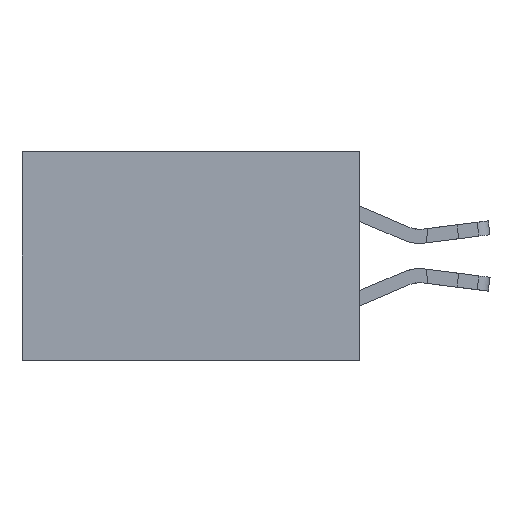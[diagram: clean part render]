
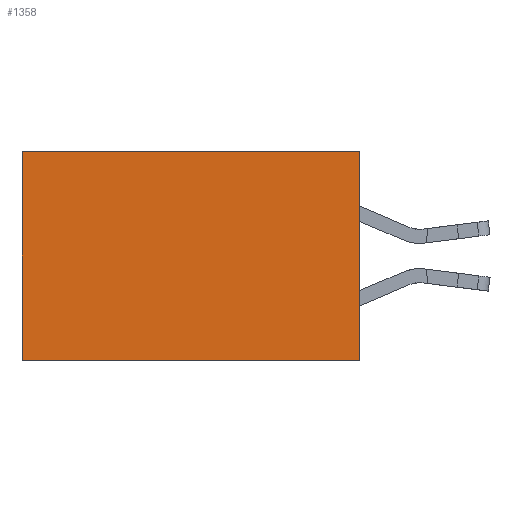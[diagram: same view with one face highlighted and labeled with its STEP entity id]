
A CAD part, left-side view. The second image highlights one B-rep face of the part: STEP entity #1358.
In plain terms, the highlighted planar face has unit normal (-1, 0, 0).
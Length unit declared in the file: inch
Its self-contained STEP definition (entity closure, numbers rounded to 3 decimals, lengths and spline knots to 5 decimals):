
#1152 = CARTESIAN_POINT ( 'NONE',  ( 0.2875, 0.6, 0. ) ) ;
#1358 = ADVANCED_FACE ( 'NONE', ( #18999 ), #18407, .F. ) ;
#1437 = CARTESIAN_POINT ( 'NONE',  ( 0.2875, 0., 0. ) ) ;
#2701 = ORIENTED_EDGE ( 'NONE', *, *, #10878, .T. ) ;
#3375 = DIRECTION ( 'NONE',  ( 0., 1., 0. ) ) ;
#4621 = VECTOR ( 'NONE', #18198, 39.37008 ) ;
#5390 = VERTEX_POINT ( 'NONE', #21293 ) ;
#5931 = CARTESIAN_POINT ( 'NONE',  ( 0.2875, 0., 0. ) ) ;
#6007 = DIRECTION ( 'NONE',  ( 0., 0., -1. ) ) ;
#7313 = ORIENTED_EDGE ( 'NONE', *, *, #21893, .F. ) ;
#7443 = VECTOR ( 'NONE', #17486, 39.37008 ) ;
#8023 = EDGE_CURVE ( 'NONE', #10039, #12910, #9150, .T. ) ;
#8754 = LINE ( 'NONE', #5931, #17206 ) ;
#9150 = LINE ( 'NONE', #1152, #4621 ) ;
#10039 = VERTEX_POINT ( 'NONE', #10046 ) ;
#10046 = CARTESIAN_POINT ( 'NONE',  ( 0.2875, 0.6, 0. ) ) ;
#10878 = EDGE_CURVE ( 'NONE', #11213, #10039, #16411, .T. ) ;
#11213 = VERTEX_POINT ( 'NONE', #19952 ) ;
#11658 = EDGE_CURVE ( 'NONE', #11213, #5390, #8754, .T. ) ;
#12512 = CARTESIAN_POINT ( 'NONE',  ( 0.2875, 0.6, -0.37 ) ) ;
#12779 = DIRECTION ( 'NONE',  ( 1., 0., 0. ) ) ;
#12910 = VERTEX_POINT ( 'NONE', #12512 ) ;
#14077 = CARTESIAN_POINT ( 'NONE',  ( 0.2875, 0., 0. ) ) ;
#14765 = ORIENTED_EDGE ( 'NONE', *, *, #8023, .T. ) ;
#15565 = AXIS2_PLACEMENT_3D ( 'NONE', #1437, #12779, #16981 ) ;
#16323 = VECTOR ( 'NONE', #3375, 39.37008 ) ;
#16411 = LINE ( 'NONE', #14077, #7443 ) ;
#16939 = CARTESIAN_POINT ( 'NONE',  ( 0.2875, 0., -0.37 ) ) ;
#16981 = DIRECTION ( 'NONE',  ( 0., 0., -1. ) ) ;
#17206 = VECTOR ( 'NONE', #6007, 39.37008 ) ;
#17392 = LINE ( 'NONE', #16939, #16323 ) ;
#17486 = DIRECTION ( 'NONE',  ( 0., 1., 0. ) ) ;
#18198 = DIRECTION ( 'NONE',  ( 0., 0., -1. ) ) ;
#18407 = PLANE ( 'NONE',  #15565 ) ;
#18999 = FACE_OUTER_BOUND ( 'NONE', #21188, .T. ) ;
#19952 = CARTESIAN_POINT ( 'NONE',  ( 0.2875, 0., 0. ) ) ;
#21188 = EDGE_LOOP ( 'NONE', ( #14765, #7313, #21588, #2701 ) ) ;
#21293 = CARTESIAN_POINT ( 'NONE',  ( 0.2875, 0., -0.37 ) ) ;
#21588 = ORIENTED_EDGE ( 'NONE', *, *, #11658, .F. ) ;
#21893 = EDGE_CURVE ( 'NONE', #5390, #12910, #17392, .T. ) ;
